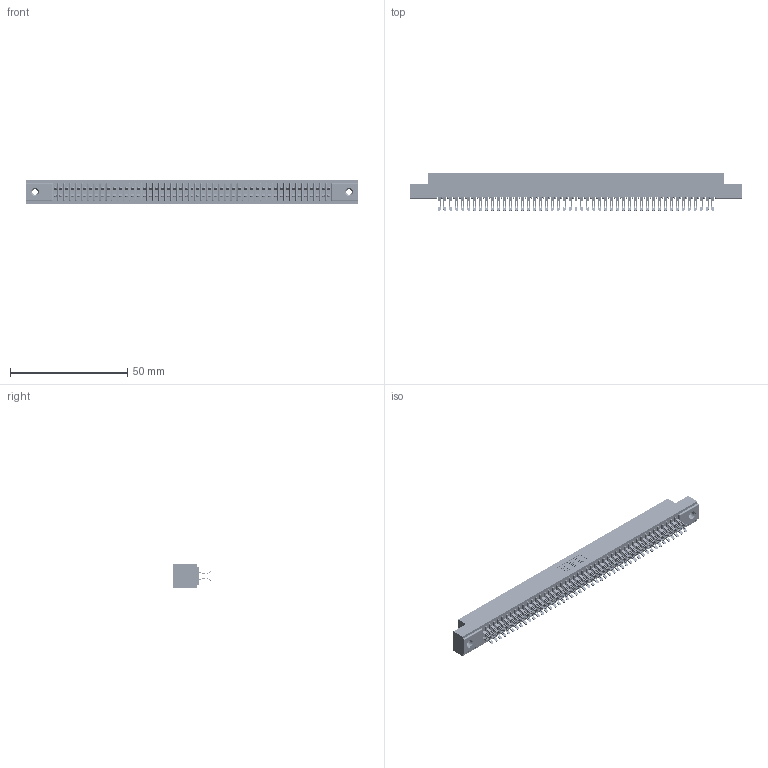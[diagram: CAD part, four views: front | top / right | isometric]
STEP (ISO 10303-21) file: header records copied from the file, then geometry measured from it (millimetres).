
FILE_DESCRIPTION (( 'STEP AP203' ), '1' );
FILE_NAME ('341-094-555-208.STEP', '2018-08-08T01:18:09', ( '' ), ( '' ), 'SwSTEP 2.0', 'SolidWorks 2016', '' );
FILE_SCHEMA (( 'CONFIG_CONTROL_DESIGN' ));
Length unit declared in the file: inch
Products named in the file (4): 341-094-555-208; 341 Part_.156 (3.96) Dia Mounting Holes; 341-292-001_341-292-155; 345-250-001_345-250-003-102
Assembly tree (97 placements, depth 2):
  341-094-555-208
    341 Part_.156 (3.96) Dia Mounting Holes
    341-292-001_341-292-155  x94
    345-250-001_345-250-003-102  x2
Bounding box: 141.6 x 16.31 x 10.16 mm (x, y, z)
Volume: 10574.2 mm3; surface area: 19714.2 mm2
Topology: 97 solids, 97 shells, 7508 faces, 22401 edges, 14578 vertices
Faces by surface type: plane 4048, cylinder 3256, sphere 96, torus 96, cone 12
Entity records: 57869 total; most frequent: CARTESIAN_POINT 9618, ORIENTED_EDGE 9542, DIRECTION 9331, EDGE_CURVE 4771, LINE 3841, VECTOR 3841, VERTEX_POINT 3016, AXIS2_PLACEMENT_3D 2745
